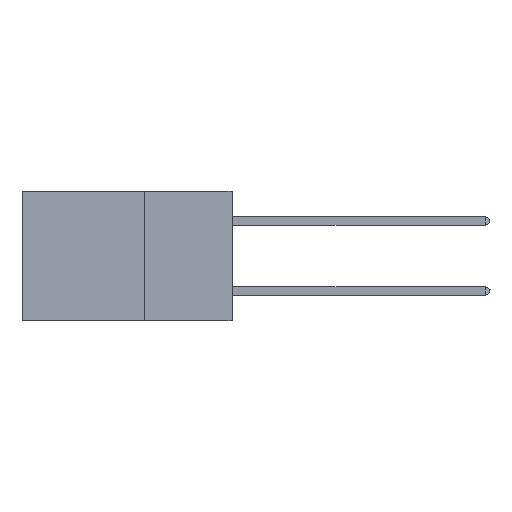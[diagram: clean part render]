
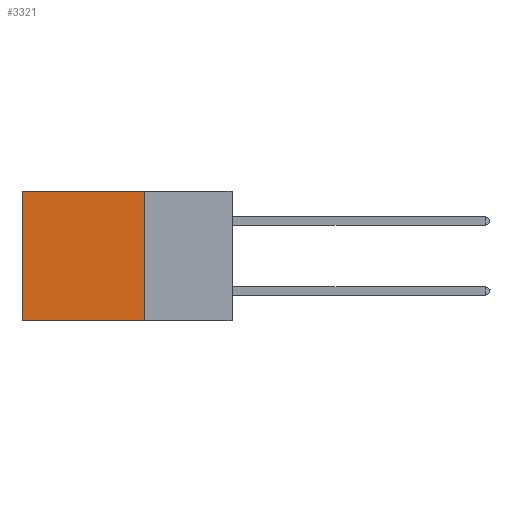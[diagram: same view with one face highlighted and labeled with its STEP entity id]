
A CAD part, left-side view. The second image highlights one B-rep face of the part: STEP entity #3321.
In plain terms, the highlighted planar face has unit normal (-1, 0, 0).
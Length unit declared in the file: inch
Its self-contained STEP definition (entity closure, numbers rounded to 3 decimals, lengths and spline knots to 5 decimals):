
#594 = AXIS2_PLACEMENT_3D ( 'NONE', #15993, #15338, #15297 ) ;
#927 = LINE ( 'NONE', #15018, #7877 ) ;
#1099 = ORIENTED_EDGE ( 'NONE', *, *, #11273, .F. ) ;
#2057 = EDGE_CURVE ( 'NONE', #6725, #17727, #14222, .T. ) ;
#3173 = VECTOR ( 'NONE', #9335, 39.37008 ) ;
#3321 = ADVANCED_FACE ( 'NONE', ( #12697 ), #17483, .F. ) ;
#3701 = DIRECTION ( 'NONE',  ( 0., 1., 0. ) ) ;
#3869 = VECTOR ( 'NONE', #17359, 39.37008 ) ;
#5428 = VECTOR ( 'NONE', #3701, 39.37008 ) ;
#6725 = VERTEX_POINT ( 'NONE', #18381 ) ;
#7709 = ORIENTED_EDGE ( 'NONE', *, *, #8761, .F. ) ;
#7877 = VECTOR ( 'NONE', #10923, 39.37008 ) ;
#8232 = LINE ( 'NONE', #16048, #3869 ) ;
#8761 = EDGE_CURVE ( 'NONE', #9012, #13471, #13550, .T. ) ;
#9012 = VERTEX_POINT ( 'NONE', #18205 ) ;
#9335 = DIRECTION ( 'NONE',  ( 0., 1., 0. ) ) ;
#9884 = CARTESIAN_POINT ( 'NONE',  ( 0.2875, 0.25, 0. ) ) ;
#10394 = CARTESIAN_POINT ( 'NONE',  ( 0.2875, 0.6, -0.37 ) ) ;
#10923 = DIRECTION ( 'NONE',  ( 0., 0., -1. ) ) ;
#10999 = CARTESIAN_POINT ( 'NONE',  ( 0.2875, 0.25, -0.37 ) ) ;
#11273 = EDGE_CURVE ( 'NONE', #6725, #9012, #927, .T. ) ;
#12664 = ORIENTED_EDGE ( 'NONE', *, *, #17562, .T. ) ;
#12697 = FACE_OUTER_BOUND ( 'NONE', #16287, .T. ) ;
#13471 = VERTEX_POINT ( 'NONE', #10394 ) ;
#13550 = LINE ( 'NONE', #10999, #5428 ) ;
#14222 = LINE ( 'NONE', #9884, #3173 ) ;
#15018 = CARTESIAN_POINT ( 'NONE',  ( 0.2875, 0.25, 0. ) ) ;
#15045 = CARTESIAN_POINT ( 'NONE',  ( 0.2875, 0.6, 0. ) ) ;
#15297 = DIRECTION ( 'NONE',  ( 0., 0., -1. ) ) ;
#15338 = DIRECTION ( 'NONE',  ( 1., 0., 0. ) ) ;
#15731 = ORIENTED_EDGE ( 'NONE', *, *, #2057, .T. ) ;
#15993 = CARTESIAN_POINT ( 'NONE',  ( 0.2875, 0.25, 0. ) ) ;
#16048 = CARTESIAN_POINT ( 'NONE',  ( 0.2875, 0.6, 0. ) ) ;
#16287 = EDGE_LOOP ( 'NONE', ( #12664, #7709, #1099, #15731 ) ) ;
#17359 = DIRECTION ( 'NONE',  ( 0., 0., -1. ) ) ;
#17483 = PLANE ( 'NONE',  #594 ) ;
#17562 = EDGE_CURVE ( 'NONE', #17727, #13471, #8232, .T. ) ;
#17727 = VERTEX_POINT ( 'NONE', #15045 ) ;
#18205 = CARTESIAN_POINT ( 'NONE',  ( 0.2875, 0.25, -0.37 ) ) ;
#18381 = CARTESIAN_POINT ( 'NONE',  ( 0.2875, 0.25, 0. ) ) ;
